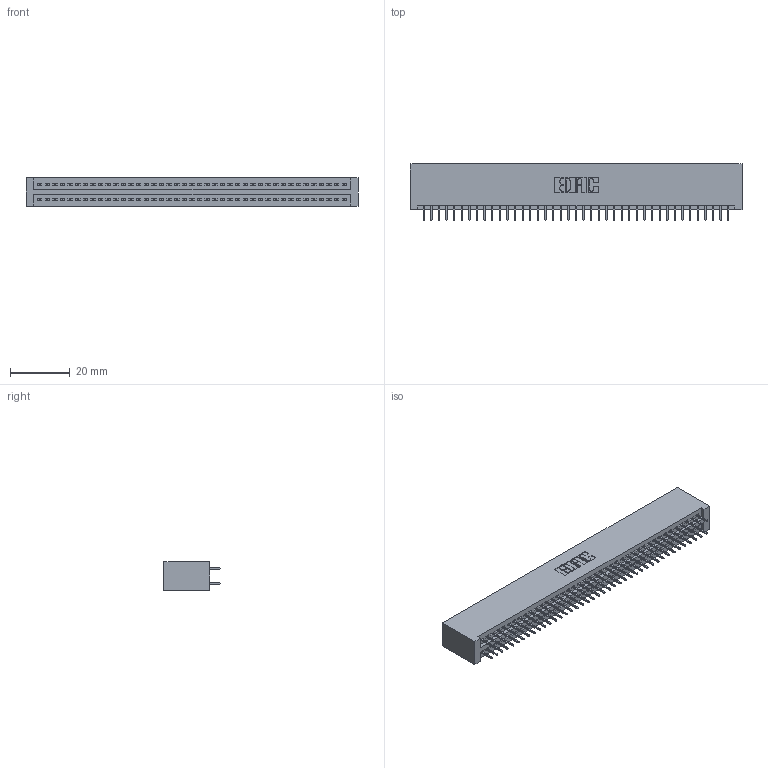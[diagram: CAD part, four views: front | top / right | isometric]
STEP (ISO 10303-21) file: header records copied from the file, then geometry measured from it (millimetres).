
FILE_DESCRIPTION (( 'STEP AP203' ), '1' );
FILE_NAME ('345-082-525-201.STEP', '2020-09-21T12:16:02', ( '' ), ( '' ), 'SwSTEP 2.0', 'SolidWorks 2020', '' );
FILE_SCHEMA (( 'CONFIG_CONTROL_DESIGN' ));
Length unit declared in the file: inch
Products named in the file (3): 345 Part_No Mounting Lugs; 345-082-525-201; 345-292-001_345-293-125
Assembly tree (83 placements, depth 2):
  345-082-525-201
    345 Part_No Mounting Lugs
    345-292-001_345-293-125  x82
Bounding box: 110.74 x 18.72 x 9.4 mm (x, y, z)
Volume: 11229.4 mm3; surface area: 16476.2 mm2
Topology: 83 solids, 83 shells, 4546 faces, 12863 edges, 8246 vertices
Faces by surface type: plane 3274, cylinder 1272
Entity records: 32101 total; most frequent: CARTESIAN_POINT 5380, ORIENTED_EDGE 5314, DIRECTION 4741, EDGE_CURVE 2657, LINE 2373, VECTOR 2373, VERTEX_POINT 1766, AXIS2_PLACEMENT_3D 1184
